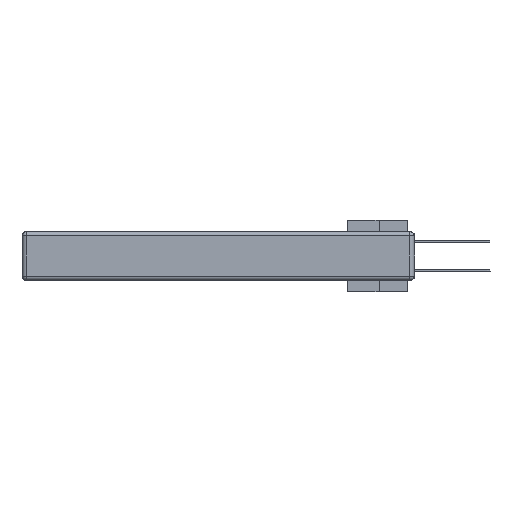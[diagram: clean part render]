
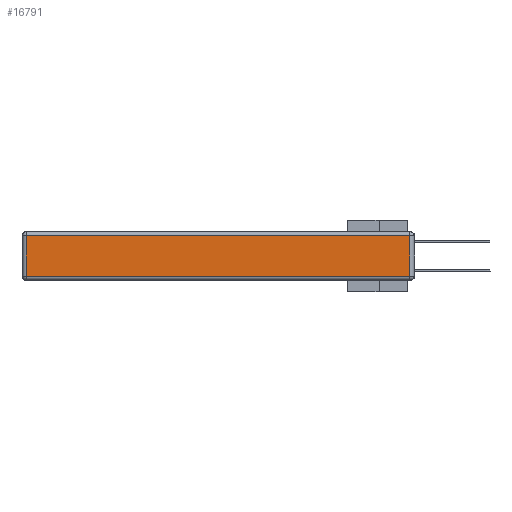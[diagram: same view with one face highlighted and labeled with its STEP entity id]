
A CAD part, left-side view. The second image highlights one B-rep face of the part: STEP entity #16791.
In plain terms, the highlighted planar face has unit normal (-1, 0, 0).
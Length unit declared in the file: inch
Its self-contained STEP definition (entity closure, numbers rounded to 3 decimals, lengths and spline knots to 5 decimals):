
#219 = ORIENTED_EDGE ( 'NONE', *, *, #27069, .T. ) ;
#1957 = CARTESIAN_POINT ( 'NONE',  ( 0., 0.03, -0.03 ) ) ;
#2214 = EDGE_LOOP ( 'NONE', ( #219, #34616, #3836, #5536 ) ) ;
#3597 = VECTOR ( 'NONE', #33348, 39.37008 ) ;
#3836 = ORIENTED_EDGE ( 'NONE', *, *, #36767, .T. ) ;
#4036 = AXIS2_PLACEMENT_3D ( 'NONE', #13347, #25000, #22704 ) ;
#4462 = VERTEX_POINT ( 'NONE', #19950 ) ;
#4564 = FACE_OUTER_BOUND ( 'NONE', #2214, .T. ) ;
#5536 = ORIENTED_EDGE ( 'NONE', *, *, #27331, .T. ) ;
#7752 = CARTESIAN_POINT ( 'NONE',  ( 0., 2.75, -0.03 ) ) ;
#8904 = CARTESIAN_POINT ( 'NONE',  ( 0., 2.72, -0.313 ) ) ;
#12277 = CARTESIAN_POINT ( 'NONE',  ( 0., 0.03, -0.313 ) ) ;
#13347 = CARTESIAN_POINT ( 'NONE',  ( 0., 0., -0.343 ) ) ;
#14245 = LINE ( 'NONE', #31298, #36563 ) ;
#15259 = DIRECTION ( 'NONE',  ( 0., -1., 0. ) ) ;
#15444 = CARTESIAN_POINT ( 'NONE',  ( 0., 0., -0.313 ) ) ;
#16266 = EDGE_CURVE ( 'NONE', #36286, #24483, #36763, .T. ) ;
#16436 = PLANE ( 'NONE',  #4036 ) ;
#16791 = ADVANCED_FACE ( 'NONE', ( #4564 ), #16436, .T. ) ;
#18014 = VECTOR ( 'NONE', #29650, 39.37008 ) ;
#19950 = CARTESIAN_POINT ( 'NONE',  ( 0., 2.72, -0.03 ) ) ;
#20680 = VECTOR ( 'NONE', #15259, 39.37008 ) ;
#22680 = DIRECTION ( 'NONE',  ( 0., 0., -1. ) ) ;
#22704 = DIRECTION ( 'NONE',  ( 0., 0., 1. ) ) ;
#24483 = VERTEX_POINT ( 'NONE', #1957 ) ;
#25000 = DIRECTION ( 'NONE',  ( -1., 0., 0. ) ) ;
#27069 = EDGE_CURVE ( 'NONE', #30001, #36286, #32654, .T. ) ;
#27331 = EDGE_CURVE ( 'NONE', #4462, #30001, #14245, .T. ) ;
#29650 = DIRECTION ( 'NONE',  ( 0., 1., 0. ) ) ;
#30001 = VERTEX_POINT ( 'NONE', #8904 ) ;
#31298 = CARTESIAN_POINT ( 'NONE',  ( 0., 2.72, -0.343 ) ) ;
#32654 = LINE ( 'NONE', #15444, #20680 ) ;
#32912 = LINE ( 'NONE', #7752, #18014 ) ;
#33155 = CARTESIAN_POINT ( 'NONE',  ( 0., 0.03, -0.343 ) ) ;
#33348 = DIRECTION ( 'NONE',  ( 0., 0., 1. ) ) ;
#34616 = ORIENTED_EDGE ( 'NONE', *, *, #16266, .T. ) ;
#36286 = VERTEX_POINT ( 'NONE', #12277 ) ;
#36563 = VECTOR ( 'NONE', #22680, 39.37008 ) ;
#36763 = LINE ( 'NONE', #33155, #3597 ) ;
#36767 = EDGE_CURVE ( 'NONE', #24483, #4462, #32912, .T. ) ;
